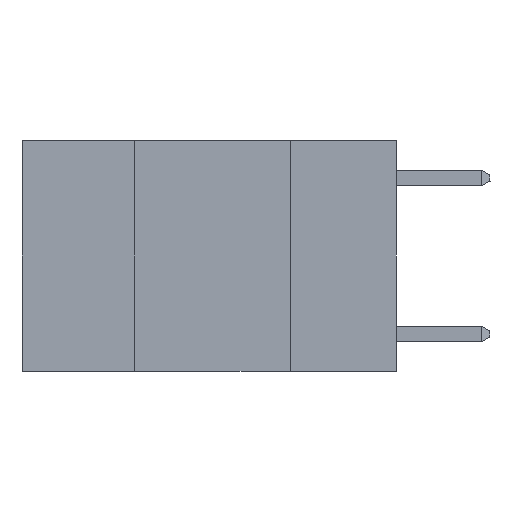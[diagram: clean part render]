
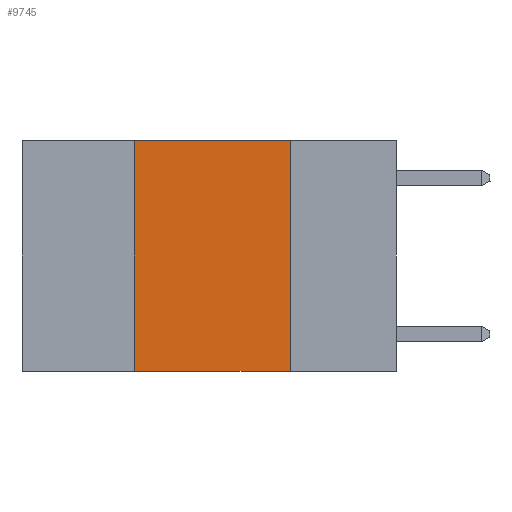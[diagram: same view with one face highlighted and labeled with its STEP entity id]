
A CAD part, left-side view. The second image highlights one B-rep face of the part: STEP entity #9745.
In plain terms, the highlighted planar face has unit normal (-1, 0, 0).
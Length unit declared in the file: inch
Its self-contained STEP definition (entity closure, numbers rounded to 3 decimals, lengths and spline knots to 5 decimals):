
#18 = CARTESIAN_POINT ( 'NONE',  ( 0., 0.17, 0. ) ) ;
#73 = ORIENTED_EDGE ( 'NONE', *, *, #1589, .T. ) ;
#954 = LINE ( 'NONE', #8374, #3872 ) ;
#985 = EDGE_CURVE ( 'NONE', #7467, #2104, #4132, .T. ) ;
#1589 = EDGE_CURVE ( 'NONE', #11759, #13708, #10993, .T. ) ;
#2104 = VERTEX_POINT ( 'NONE', #18 ) ;
#2545 = ORIENTED_EDGE ( 'NONE', *, *, #5776, .F. ) ;
#2895 = DIRECTION ( 'NONE',  ( 0., 0., -1. ) ) ;
#3073 = EDGE_CURVE ( 'NONE', #2104, #13708, #954, .T. ) ;
#3872 = VECTOR ( 'NONE', #2895, 39.37008 ) ;
#4037 = CARTESIAN_POINT ( 'NONE',  ( 0., 0.17, -0.37 ) ) ;
#4132 = LINE ( 'NONE', #8786, #7351 ) ;
#4145 = FACE_OUTER_BOUND ( 'NONE', #11427, .T. ) ;
#4349 = DIRECTION ( 'NONE',  ( 0., -1., 0. ) ) ;
#4395 = VECTOR ( 'NONE', #9241, 39.37008 ) ;
#4704 = PLANE ( 'NONE',  #7489 ) ;
#5776 = EDGE_CURVE ( 'NONE', #11759, #7467, #7585, .T. ) ;
#5850 = CARTESIAN_POINT ( 'NONE',  ( 0., 0.42, 0. ) ) ;
#5928 = DIRECTION ( 'NONE',  ( 1., 0., 0. ) ) ;
#6046 = ORIENTED_EDGE ( 'NONE', *, *, #3073, .F. ) ;
#6809 = CARTESIAN_POINT ( 'NONE',  ( 0., 0.42, -0.37 ) ) ;
#7351 = VECTOR ( 'NONE', #4349, 39.37008 ) ;
#7467 = VERTEX_POINT ( 'NONE', #5850 ) ;
#7489 = AXIS2_PLACEMENT_3D ( 'NONE', #13257, #5928, #14365 ) ;
#7585 = LINE ( 'NONE', #7984, #4395 ) ;
#7698 = VECTOR ( 'NONE', #14637, 39.37008 ) ;
#7984 = CARTESIAN_POINT ( 'NONE',  ( 0., 0.42, 0. ) ) ;
#8374 = CARTESIAN_POINT ( 'NONE',  ( 0., 0.17, 0. ) ) ;
#8786 = CARTESIAN_POINT ( 'NONE',  ( 0., 0.6, 0. ) ) ;
#9241 = DIRECTION ( 'NONE',  ( 0., 0., 1. ) ) ;
#9745 = ADVANCED_FACE ( 'NONE', ( #4145 ), #4704, .F. ) ;
#10993 = LINE ( 'NONE', #11336, #7698 ) ;
#11336 = CARTESIAN_POINT ( 'NONE',  ( 0., 0.6, -0.37 ) ) ;
#11427 = EDGE_LOOP ( 'NONE', ( #6046, #13954, #2545, #73 ) ) ;
#11759 = VERTEX_POINT ( 'NONE', #6809 ) ;
#13257 = CARTESIAN_POINT ( 'NONE',  ( 0., 0.6, 0. ) ) ;
#13708 = VERTEX_POINT ( 'NONE', #4037 ) ;
#13954 = ORIENTED_EDGE ( 'NONE', *, *, #985, .F. ) ;
#14365 = DIRECTION ( 'NONE',  ( 0., 0., -1. ) ) ;
#14637 = DIRECTION ( 'NONE',  ( 0., -1., 0. ) ) ;
